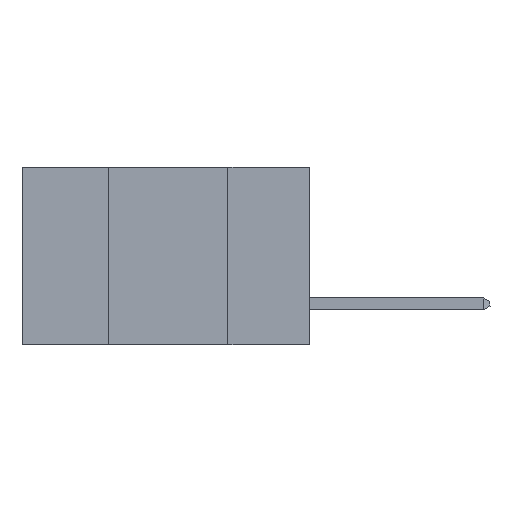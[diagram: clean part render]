
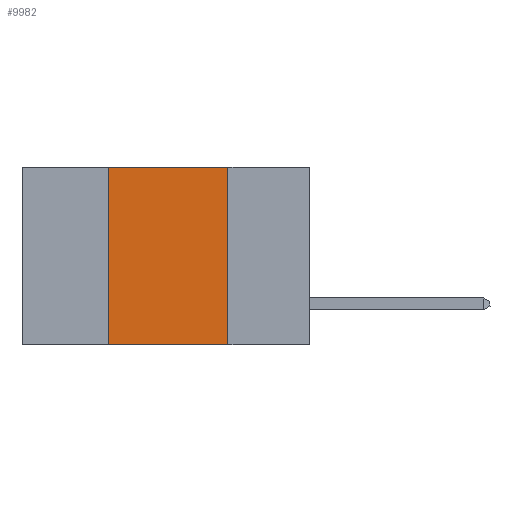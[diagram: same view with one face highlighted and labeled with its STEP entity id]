
A CAD part, left-side view. The second image highlights one B-rep face of the part: STEP entity #9982.
In plain terms, the highlighted planar face has unit normal (-1, 0, 0).
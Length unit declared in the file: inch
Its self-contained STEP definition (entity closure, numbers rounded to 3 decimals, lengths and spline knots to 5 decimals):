
#603 = ORIENTED_EDGE ( 'NONE', *, *, #9410, .T. ) ;
#807 = VERTEX_POINT ( 'NONE', #9117 ) ;
#1169 = VERTEX_POINT ( 'NONE', #9585 ) ;
#1933 = CARTESIAN_POINT ( 'NONE',  ( 0., 0.6, -0.37 ) ) ;
#1941 = VECTOR ( 'NONE', #7562, 39.37008 ) ;
#1956 = VECTOR ( 'NONE', #10065, 39.37008 ) ;
#2354 = VERTEX_POINT ( 'NONE', #10181 ) ;
#2898 = VECTOR ( 'NONE', #11046, 39.37008 ) ;
#3159 = ORIENTED_EDGE ( 'NONE', *, *, #5488, .F. ) ;
#3387 = EDGE_LOOP ( 'NONE', ( #7729, #3159, #6001, #603 ) ) ;
#3574 = VERTEX_POINT ( 'NONE', #3781 ) ;
#3781 = CARTESIAN_POINT ( 'NONE',  ( 0., 0.42, 0. ) ) ;
#4123 = EDGE_CURVE ( 'NONE', #2354, #807, #10855, .T. ) ;
#5145 = LINE ( 'NONE', #1933, #9485 ) ;
#5186 = PLANE ( 'NONE',  #7518 ) ;
#5239 = LINE ( 'NONE', #11285, #2898 ) ;
#5488 = EDGE_CURVE ( 'NONE', #3574, #2354, #5239, .T. ) ;
#6001 = ORIENTED_EDGE ( 'NONE', *, *, #7835, .F. ) ;
#6095 = DIRECTION ( 'NONE',  ( 0., 0., -1. ) ) ;
#6399 = DIRECTION ( 'NONE',  ( 0., -1., 0. ) ) ;
#7510 = CARTESIAN_POINT ( 'NONE',  ( 0., 0.17, 0. ) ) ;
#7518 = AXIS2_PLACEMENT_3D ( 'NONE', #9507, #11100, #6095 ) ;
#7562 = DIRECTION ( 'NONE',  ( 0., 0., -1. ) ) ;
#7729 = ORIENTED_EDGE ( 'NONE', *, *, #4123, .F. ) ;
#7835 = EDGE_CURVE ( 'NONE', #1169, #3574, #10620, .T. ) ;
#9117 = CARTESIAN_POINT ( 'NONE',  ( 0., 0.17, -0.37 ) ) ;
#9410 = EDGE_CURVE ( 'NONE', #1169, #807, #5145, .T. ) ;
#9485 = VECTOR ( 'NONE', #6399, 39.37008 ) ;
#9507 = CARTESIAN_POINT ( 'NONE',  ( 0., 0.6, 0. ) ) ;
#9585 = CARTESIAN_POINT ( 'NONE',  ( 0., 0.42, -0.37 ) ) ;
#9982 = ADVANCED_FACE ( 'NONE', ( #10339 ), #5186, .F. ) ;
#10065 = DIRECTION ( 'NONE',  ( 0., 0., 1. ) ) ;
#10103 = CARTESIAN_POINT ( 'NONE',  ( 0., 0.42, 0. ) ) ;
#10181 = CARTESIAN_POINT ( 'NONE',  ( 0., 0.17, 0. ) ) ;
#10339 = FACE_OUTER_BOUND ( 'NONE', #3387, .T. ) ;
#10620 = LINE ( 'NONE', #10103, #1956 ) ;
#10855 = LINE ( 'NONE', #7510, #1941 ) ;
#11046 = DIRECTION ( 'NONE',  ( 0., -1., 0. ) ) ;
#11100 = DIRECTION ( 'NONE',  ( 1., 0., 0. ) ) ;
#11285 = CARTESIAN_POINT ( 'NONE',  ( 0., 0.6, 0. ) ) ;
